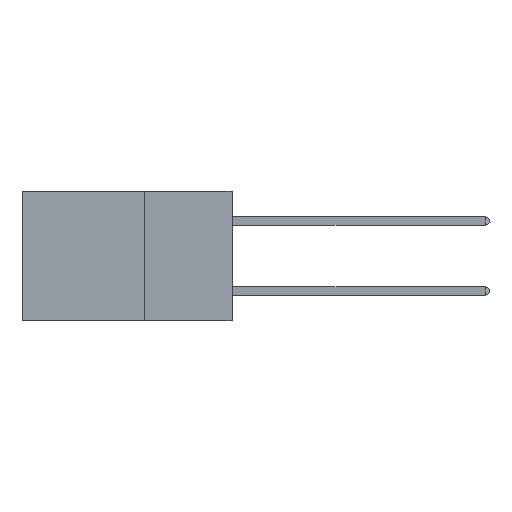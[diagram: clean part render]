
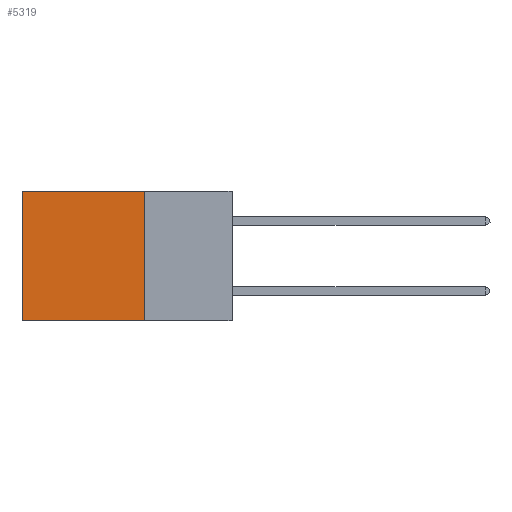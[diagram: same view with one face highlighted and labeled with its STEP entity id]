
A CAD part, left-side view. The second image highlights one B-rep face of the part: STEP entity #5319.
In plain terms, the highlighted planar face has unit normal (-1, 0, 0).
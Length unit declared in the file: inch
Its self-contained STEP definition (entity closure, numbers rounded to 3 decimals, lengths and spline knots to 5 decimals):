
#2351 = VECTOR ( 'NONE', #6920, 39.37008 ) ;
#2393 = CARTESIAN_POINT ( 'NONE',  ( 0.2875, 0.25, 0. ) ) ;
#2924 = AXIS2_PLACEMENT_3D ( 'NONE', #13499, #16375, #7022 ) ;
#3355 = CARTESIAN_POINT ( 'NONE',  ( 0.2875, 0.25, -0.37 ) ) ;
#5319 = ADVANCED_FACE ( 'NONE', ( #14045 ), #5417, .F. ) ;
#5417 = PLANE ( 'NONE',  #2924 ) ;
#5568 = VERTEX_POINT ( 'NONE', #19075 ) ;
#5596 = LINE ( 'NONE', #17773, #2351 ) ;
#5613 = LINE ( 'NONE', #20393, #18136 ) ;
#6641 = DIRECTION ( 'NONE',  ( 0., 0., -1. ) ) ;
#6920 = DIRECTION ( 'NONE',  ( 0., 0., -1. ) ) ;
#7022 = DIRECTION ( 'NONE',  ( 0., 0., -1. ) ) ;
#7593 = VECTOR ( 'NONE', #6641, 39.37008 ) ;
#7620 = DIRECTION ( 'NONE',  ( 0., 1., 0. ) ) ;
#12275 = ORIENTED_EDGE ( 'NONE', *, *, #12944, .T. ) ;
#12944 = EDGE_CURVE ( 'NONE', #15289, #5568, #14955, .T. ) ;
#13032 = CARTESIAN_POINT ( 'NONE',  ( 0.2875, 0.25, 0. ) ) ;
#13065 = EDGE_CURVE ( 'NONE', #14778, #15220, #5613, .T. ) ;
#13499 = CARTESIAN_POINT ( 'NONE',  ( 0.2875, 0.25, 0. ) ) ;
#13652 = EDGE_CURVE ( 'NONE', #5568, #15220, #5596, .T. ) ;
#13656 = EDGE_CURVE ( 'NONE', #15289, #14778, #16623, .T. ) ;
#14045 = FACE_OUTER_BOUND ( 'NONE', #18370, .T. ) ;
#14227 = VECTOR ( 'NONE', #7620, 39.37008 ) ;
#14778 = VERTEX_POINT ( 'NONE', #3355 ) ;
#14955 = LINE ( 'NONE', #2393, #14227 ) ;
#15220 = VERTEX_POINT ( 'NONE', #19311 ) ;
#15289 = VERTEX_POINT ( 'NONE', #16170 ) ;
#16170 = CARTESIAN_POINT ( 'NONE',  ( 0.2875, 0.25, 0. ) ) ;
#16375 = DIRECTION ( 'NONE',  ( 1., 0., 0. ) ) ;
#16623 = LINE ( 'NONE', #13032, #7593 ) ;
#16643 = ORIENTED_EDGE ( 'NONE', *, *, #13652, .T. ) ;
#17773 = CARTESIAN_POINT ( 'NONE',  ( 0.2875, 0.6, 0. ) ) ;
#18136 = VECTOR ( 'NONE', #18611, 39.37008 ) ;
#18370 = EDGE_LOOP ( 'NONE', ( #16643, #20264, #19815, #12275 ) ) ;
#18611 = DIRECTION ( 'NONE',  ( 0., 1., 0. ) ) ;
#19075 = CARTESIAN_POINT ( 'NONE',  ( 0.2875, 0.6, 0. ) ) ;
#19311 = CARTESIAN_POINT ( 'NONE',  ( 0.2875, 0.6, -0.37 ) ) ;
#19815 = ORIENTED_EDGE ( 'NONE', *, *, #13656, .F. ) ;
#20264 = ORIENTED_EDGE ( 'NONE', *, *, #13065, .F. ) ;
#20393 = CARTESIAN_POINT ( 'NONE',  ( 0.2875, 0.25, -0.37 ) ) ;
